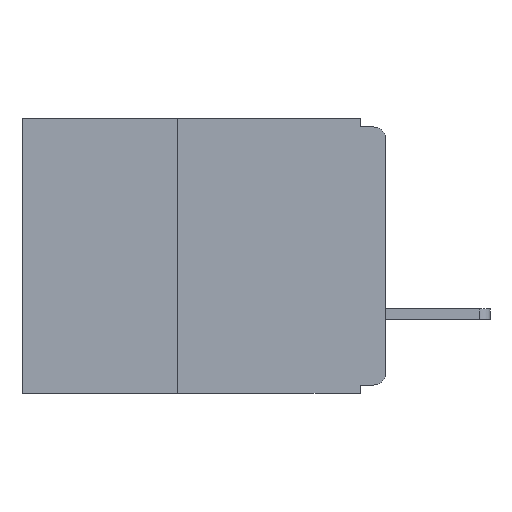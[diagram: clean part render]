
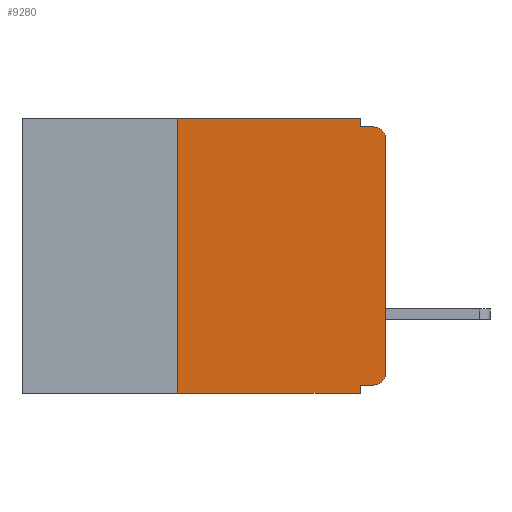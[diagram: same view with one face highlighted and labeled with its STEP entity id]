
A CAD part, left-side view. The second image highlights one B-rep face of the part: STEP entity #9280.
In plain terms, the highlighted planar face has unit normal (-1, 0, 0).
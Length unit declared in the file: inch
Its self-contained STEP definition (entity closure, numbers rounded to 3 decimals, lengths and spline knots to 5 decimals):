
#474 = AXIS2_PLACEMENT_3D ( 'NONE', #6933, #6870, #6843 ) ;
#656 = CARTESIAN_POINT ( 'NONE',  ( 0., 0., -0.305 ) ) ;
#750 = CARTESIAN_POINT ( 'NONE',  ( 0., 0.031, -0.33 ) ) ;
#790 = ORIENTED_EDGE ( 'NONE', *, *, #7721, .F. ) ;
#858 = LINE ( 'NONE', #13164, #13855 ) ;
#1544 = LINE ( 'NONE', #9720, #7701 ) ;
#1734 = VERTEX_POINT ( 'NONE', #656 ) ;
#1958 = AXIS2_PLACEMENT_3D ( 'NONE', #6928, #6858, #6837 ) ;
#2167 = CARTESIAN_POINT ( 'NONE',  ( 0., 0.015, -0.32 ) ) ;
#2369 = DIRECTION ( 'NONE',  ( 0., 0., 1. ) ) ;
#2531 = LINE ( 'NONE', #6199, #15157 ) ;
#3037 = VERTEX_POINT ( 'NONE', #7093 ) ;
#3051 = CIRCLE ( 'NONE', #11282, 0.015 ) ;
#3375 = DIRECTION ( 'NONE',  ( 0., -1., 0. ) ) ;
#3640 = VERTEX_POINT ( 'NONE', #750 ) ;
#4355 = VERTEX_POINT ( 'NONE', #7500 ) ;
#4646 = VERTEX_POINT ( 'NONE', #2167 ) ;
#4699 = ORIENTED_EDGE ( 'NONE', *, *, #5750, .T. ) ;
#4851 = VERTEX_POINT ( 'NONE', #15451 ) ;
#4862 = VERTEX_POINT ( 'NONE', #16008 ) ;
#5090 = EDGE_CURVE ( 'NONE', #1734, #4862, #858, .T. ) ;
#5121 = ORIENTED_EDGE ( 'NONE', *, *, #5090, .T. ) ;
#5327 = EDGE_CURVE ( 'NONE', #11733, #11473, #9521, .T. ) ;
#5582 = VECTOR ( 'NONE', #3375, 39.37008 ) ;
#5613 = EDGE_CURVE ( 'NONE', #4646, #3037, #1544, .T. ) ;
#5641 = VERTEX_POINT ( 'NONE', #9378 ) ;
#5660 = EDGE_CURVE ( 'NONE', #4862, #11473, #3051, .T. ) ;
#5719 = ORIENTED_EDGE ( 'NONE', *, *, #7798, .F. ) ;
#5734 = ORIENTED_EDGE ( 'NONE', *, *, #5660, .T. ) ;
#5750 = EDGE_CURVE ( 'NONE', #4646, #1734, #8318, .T. ) ;
#5967 = LINE ( 'NONE', #15483, #5582 ) ;
#6055 = DIRECTION ( 'NONE',  ( 0., 0., -1. ) ) ;
#6199 = CARTESIAN_POINT ( 'NONE',  ( 0., 0.031, -0.33 ) ) ;
#6434 = DIRECTION ( 'NONE',  ( 0., -1., 0. ) ) ;
#6489 = CARTESIAN_POINT ( 'NONE',  ( 0., 0.437, -0.33 ) ) ;
#6754 = DIRECTION ( 'NONE',  ( 0., 0., 1. ) ) ;
#6767 = CARTESIAN_POINT ( 'NONE',  ( 0., 0.25, -0.33 ) ) ;
#6837 = DIRECTION ( 'NONE',  ( 0., 0., -1. ) ) ;
#6843 = DIRECTION ( 'NONE',  ( 0., 0., -1. ) ) ;
#6858 = DIRECTION ( 'NONE',  ( 1., 0., 0. ) ) ;
#6870 = DIRECTION ( 'NONE',  ( -1., 0., 0. ) ) ;
#6928 = CARTESIAN_POINT ( 'NONE',  ( 0., 0.437, 0. ) ) ;
#6933 = CARTESIAN_POINT ( 'NONE',  ( 0., 0.015, -0.305 ) ) ;
#6943 = DIRECTION ( 'NONE',  ( 0., 0., -1. ) ) ;
#6955 = PLANE ( 'NONE',  #1958 ) ;
#7008 = CARTESIAN_POINT ( 'NONE',  ( 0., 0.031, 0. ) ) ;
#7045 = ORIENTED_EDGE ( 'NONE', *, *, #5613, .F. ) ;
#7093 = CARTESIAN_POINT ( 'NONE',  ( 0., 0.031, -0.32 ) ) ;
#7210 = VECTOR ( 'NONE', #6754, 39.37008 ) ;
#7263 = ORIENTED_EDGE ( 'NONE', *, *, #5327, .F. ) ;
#7351 = FACE_OUTER_BOUND ( 'NONE', #14537, .T. ) ;
#7500 = CARTESIAN_POINT ( 'NONE',  ( 0., 0.25, 0. ) ) ;
#7600 = ORIENTED_EDGE ( 'NONE', *, *, #7695, .F. ) ;
#7613 = VECTOR ( 'NONE', #6943, 39.37008 ) ;
#7695 = EDGE_CURVE ( 'NONE', #5641, #11733, #13943, .T. ) ;
#7701 = VECTOR ( 'NONE', #9469, 39.37008 ) ;
#7721 = EDGE_CURVE ( 'NONE', #4851, #4355, #13609, .T. ) ;
#7774 = EDGE_CURVE ( 'NONE', #4851, #3640, #9800, .T. ) ;
#7798 = EDGE_CURVE ( 'NONE', #3037, #3640, #2531, .T. ) ;
#8224 = CARTESIAN_POINT ( 'NONE',  ( 0., 0.031, -0.01 ) ) ;
#8318 = CIRCLE ( 'NONE', #474, 0.015 ) ;
#8364 = DIRECTION ( 'NONE',  ( 0., 0., -1. ) ) ;
#8374 = DIRECTION ( 'NONE',  ( -1., 0., 0. ) ) ;
#8412 = CARTESIAN_POINT ( 'NONE',  ( 0., 0.015, -0.025 ) ) ;
#8795 = ORIENTED_EDGE ( 'NONE', *, *, #7774, .T. ) ;
#9280 = ADVANCED_FACE ( 'NONE', ( #7351 ), #6955, .F. ) ;
#9378 = CARTESIAN_POINT ( 'NONE',  ( 0., 0.031, 0. ) ) ;
#9469 = DIRECTION ( 'NONE',  ( 0., 1., 0. ) ) ;
#9521 = LINE ( 'NONE', #13498, #13008 ) ;
#9720 = CARTESIAN_POINT ( 'NONE',  ( 0., 0., -0.32 ) ) ;
#9800 = LINE ( 'NONE', #6489, #15796 ) ;
#11282 = AXIS2_PLACEMENT_3D ( 'NONE', #8412, #8374, #8364 ) ;
#11473 = VERTEX_POINT ( 'NONE', #15864 ) ;
#11733 = VERTEX_POINT ( 'NONE', #8224 ) ;
#13008 = VECTOR ( 'NONE', #13410, 39.37008 ) ;
#13164 = CARTESIAN_POINT ( 'NONE',  ( 0., 0., 0. ) ) ;
#13410 = DIRECTION ( 'NONE',  ( 0., -1., 0. ) ) ;
#13498 = CARTESIAN_POINT ( 'NONE',  ( 0., 0., -0.01 ) ) ;
#13609 = LINE ( 'NONE', #6767, #7210 ) ;
#13855 = VECTOR ( 'NONE', #2369, 39.37008 ) ;
#13943 = LINE ( 'NONE', #7008, #7613 ) ;
#14435 = ORIENTED_EDGE ( 'NONE', *, *, #14560, .F. ) ;
#14537 = EDGE_LOOP ( 'NONE', ( #5121, #5734, #7263, #7600, #14435, #790, #8795, #5719, #7045, #4699 ) ) ;
#14560 = EDGE_CURVE ( 'NONE', #4355, #5641, #5967, .T. ) ;
#15157 = VECTOR ( 'NONE', #6055, 39.37008 ) ;
#15451 = CARTESIAN_POINT ( 'NONE',  ( 0., 0.25, -0.33 ) ) ;
#15483 = CARTESIAN_POINT ( 'NONE',  ( 0., 0.437, 0. ) ) ;
#15796 = VECTOR ( 'NONE', #6434, 39.37008 ) ;
#15864 = CARTESIAN_POINT ( 'NONE',  ( 0., 0.015, -0.01 ) ) ;
#16008 = CARTESIAN_POINT ( 'NONE',  ( 0., 0., -0.025 ) ) ;
